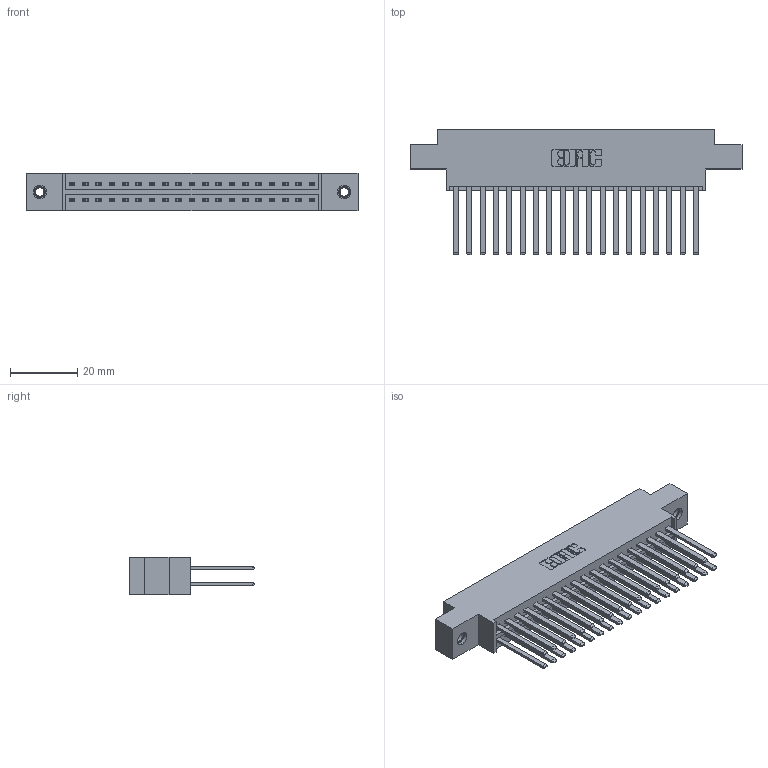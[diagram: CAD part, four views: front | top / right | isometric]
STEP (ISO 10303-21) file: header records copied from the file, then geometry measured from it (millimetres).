
FILE_DESCRIPTION (( 'STEP AP203' ), '1' );
FILE_NAME ('336-038-541-807.STEP', '2020-08-07T23:05:53', ( '' ), ( '' ), 'SwSTEP 2.0', 'SolidWorks 2020', '' );
FILE_SCHEMA (( 'CONFIG_CONTROL_DESIGN' ));
Length unit declared in the file: inch
Products named in the file (4): 336 Part_Offset - .156 Dia - TI; 336-038-541-807; 345-250-001_345-250-005-103; 336-290-001_336-290-541
Assembly tree (41 placements, depth 2):
  336-038-541-807
    336 Part_Offset - .156 Dia - TI
    336-290-001_336-290-541  x38
    345-250-001_345-250-005-103  x2
Bounding box: 98.68 x 37.34 x 11.1 mm (x, y, z)
Volume: 14469.3 mm3; surface area: 18141.3 mm2
Topology: 41 solids, 41 shells, 1774 faces, 5285 edges, 3490 vertices
Faces by surface type: plane 1094, cylinder 664, cone 12, torus 4
Entity records: 18743 total; most frequent: CARTESIAN_POINT 3240, ORIENTED_EDGE 3070, DIRECTION 2733, EDGE_CURVE 1535, VECTOR 1383, LINE 1383, VERTEX_POINT 1018, AXIS2_PLACEMENT_3D 675
